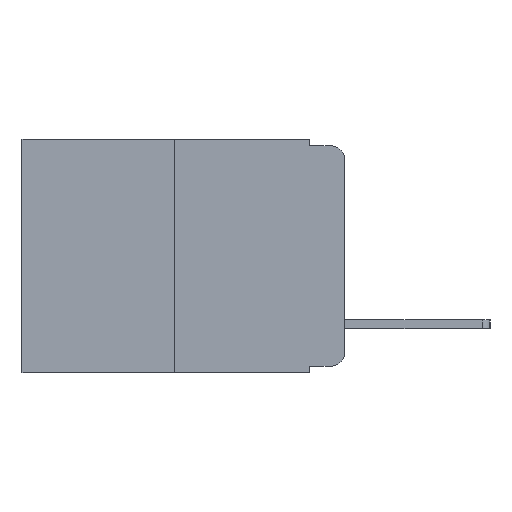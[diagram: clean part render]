
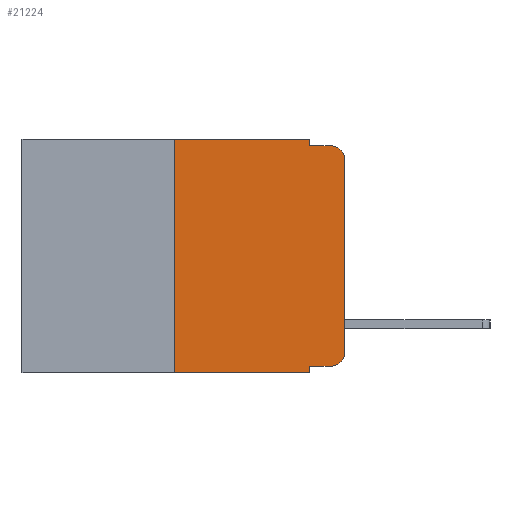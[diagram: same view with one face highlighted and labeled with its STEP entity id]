
A CAD part, left-side view. The second image highlights one B-rep face of the part: STEP entity #21224.
In plain terms, the highlighted planar face has unit normal (-1, 0, 0).
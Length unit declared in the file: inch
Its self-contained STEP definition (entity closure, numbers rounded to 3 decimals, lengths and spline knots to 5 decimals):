
#1038 = VERTEX_POINT ( 'NONE', #17887 ) ;
#1089 = VERTEX_POINT ( 'NONE', #10230 ) ;
#1184 = EDGE_CURVE ( 'NONE', #1038, #3285, #2464, .T. ) ;
#1366 = VERTEX_POINT ( 'NONE', #21364 ) ;
#1428 = EDGE_LOOP ( 'NONE', ( #6493, #21380, #1842, #4576, #2442, #1454, #11451, #9322, #11807, #7376 ) ) ;
#1454 = ORIENTED_EDGE ( 'NONE', *, *, #2565, .F. ) ;
#1701 = CIRCLE ( 'NONE', #21722, 0.02 ) ;
#1842 = ORIENTED_EDGE ( 'NONE', *, *, #2498, .F. ) ;
#1847 = EDGE_CURVE ( 'NONE', #9586, #7723, #10729, .T. ) ;
#2425 = EDGE_CURVE ( 'NONE', #1366, #1089, #13126, .T. ) ;
#2428 = EDGE_CURVE ( 'NONE', #1089, #21960, #3283, .T. ) ;
#2442 = ORIENTED_EDGE ( 'NONE', *, *, #1184, .F. ) ;
#2464 = LINE ( 'NONE', #22741, #12940 ) ;
#2498 = EDGE_CURVE ( 'NONE', #7603, #21960, #6714, .T. ) ;
#2534 = EDGE_CURVE ( 'NONE', #3285, #7603, #14385, .T. ) ;
#2565 = EDGE_CURVE ( 'NONE', #9586, #1038, #3569, .T. ) ;
#2567 = EDGE_CURVE ( 'NONE', #15228, #7723, #12837, .T. ) ;
#2607 = EDGE_CURVE ( 'NONE', #15228, #16718, #13386, .T. ) ;
#2643 = EDGE_CURVE ( 'NONE', #16718, #1366, #1701, .T. ) ;
#2973 = VECTOR ( 'NONE', #13992, 39.37008 ) ;
#3014 = DIRECTION ( 'NONE',  ( 0., 0., -1. ) ) ;
#3036 = AXIS2_PLACEMENT_3D ( 'NONE', #14989, #4194, #16692 ) ;
#3182 = DIRECTION ( 'NONE',  ( 0., -1., 0. ) ) ;
#3283 = CIRCLE ( 'NONE', #3036, 0.02 ) ;
#3285 = VERTEX_POINT ( 'NONE', #9413 ) ;
#3569 = LINE ( 'NONE', #15731, #17275 ) ;
#3944 = CARTESIAN_POINT ( 'NONE',  ( 0., 0.051, -0.343 ) ) ;
#3956 = DIRECTION ( 'NONE',  ( 0., -1., 0. ) ) ;
#4105 = DIRECTION ( 'NONE',  ( 0., 0., 1. ) ) ;
#4194 = DIRECTION ( 'NONE',  ( -1., 0., 0. ) ) ;
#4576 = ORIENTED_EDGE ( 'NONE', *, *, #2534, .F. ) ;
#5427 = VECTOR ( 'NONE', #18516, 39.37008 ) ;
#6493 = ORIENTED_EDGE ( 'NONE', *, *, #2425, .T. ) ;
#6714 = LINE ( 'NONE', #12219, #5427 ) ;
#7376 = ORIENTED_EDGE ( 'NONE', *, *, #2643, .T. ) ;
#7422 = CARTESIAN_POINT ( 'NONE',  ( 0., 0.02, -0.313 ) ) ;
#7603 = VERTEX_POINT ( 'NONE', #9153 ) ;
#7723 = VERTEX_POINT ( 'NONE', #3944 ) ;
#8448 = CARTESIAN_POINT ( 'NONE',  ( 0., 0.02, -0.333 ) ) ;
#8639 = FACE_OUTER_BOUND ( 'NONE', #1428, .T. ) ;
#9153 = CARTESIAN_POINT ( 'NONE',  ( 0., 0.051, -0.01 ) ) ;
#9285 = DIRECTION ( 'NONE',  ( 0., 0., -1. ) ) ;
#9322 = ORIENTED_EDGE ( 'NONE', *, *, #2567, .F. ) ;
#9349 = VECTOR ( 'NONE', #3014, 39.37008 ) ;
#9413 = CARTESIAN_POINT ( 'NONE',  ( 0., 0.051, 0. ) ) ;
#9586 = VERTEX_POINT ( 'NONE', #14764 ) ;
#10230 = CARTESIAN_POINT ( 'NONE',  ( 0., 0., -0.03 ) ) ;
#10495 = DIRECTION ( 'NONE',  ( 0., 0., -1. ) ) ;
#10729 = LINE ( 'NONE', #13162, #22814 ) ;
#10881 = DIRECTION ( 'NONE',  ( 0., -1., 0. ) ) ;
#11043 = CARTESIAN_POINT ( 'NONE',  ( 0., 0.051, -0.333 ) ) ;
#11451 = ORIENTED_EDGE ( 'NONE', *, *, #1847, .T. ) ;
#11807 = ORIENTED_EDGE ( 'NONE', *, *, #2607, .T. ) ;
#12219 = CARTESIAN_POINT ( 'NONE',  ( 0., 0.051, -0.01 ) ) ;
#12837 = LINE ( 'NONE', #22174, #2973 ) ;
#12940 = VECTOR ( 'NONE', #3182, 39.37008 ) ;
#13126 = LINE ( 'NONE', #18239, #17032 ) ;
#13162 = CARTESIAN_POINT ( 'NONE',  ( 0., 0.473, -0.343 ) ) ;
#13386 = LINE ( 'NONE', #19127, #16234 ) ;
#13992 = DIRECTION ( 'NONE',  ( 0., 0., -1. ) ) ;
#14344 = CARTESIAN_POINT ( 'NONE',  ( 0., 0.02, -0.01 ) ) ;
#14385 = LINE ( 'NONE', #20501, #9349 ) ;
#14764 = CARTESIAN_POINT ( 'NONE',  ( 0., 0.25, -0.343 ) ) ;
#14989 = CARTESIAN_POINT ( 'NONE',  ( 0., 0.02, -0.03 ) ) ;
#15228 = VERTEX_POINT ( 'NONE', #11043 ) ;
#15731 = CARTESIAN_POINT ( 'NONE',  ( 0., 0.25, 0. ) ) ;
#16234 = VECTOR ( 'NONE', #10881, 39.37008 ) ;
#16692 = DIRECTION ( 'NONE',  ( 0., 0., -1. ) ) ;
#16718 = VERTEX_POINT ( 'NONE', #8448 ) ;
#17032 = VECTOR ( 'NONE', #4105, 39.37008 ) ;
#17275 = VECTOR ( 'NONE', #17395, 39.37008 ) ;
#17395 = DIRECTION ( 'NONE',  ( 0., 0., 1. ) ) ;
#17887 = CARTESIAN_POINT ( 'NONE',  ( 0., 0.25, 0. ) ) ;
#17923 = AXIS2_PLACEMENT_3D ( 'NONE', #20246, #20391, #10495 ) ;
#18239 = CARTESIAN_POINT ( 'NONE',  ( 0., 0., 0. ) ) ;
#18516 = DIRECTION ( 'NONE',  ( 0., -1., 0. ) ) ;
#18760 = PLANE ( 'NONE',  #17923 ) ;
#19127 = CARTESIAN_POINT ( 'NONE',  ( 0., 0.051, -0.333 ) ) ;
#19269 = DIRECTION ( 'NONE',  ( -1., 0., 0. ) ) ;
#20246 = CARTESIAN_POINT ( 'NONE',  ( 0., 0.473, 0. ) ) ;
#20391 = DIRECTION ( 'NONE',  ( 1., 0., 0. ) ) ;
#20501 = CARTESIAN_POINT ( 'NONE',  ( 0., 0.051, 0. ) ) ;
#21224 = ADVANCED_FACE ( 'NONE', ( #8639 ), #18760, .F. ) ;
#21364 = CARTESIAN_POINT ( 'NONE',  ( 0., 0., -0.313 ) ) ;
#21380 = ORIENTED_EDGE ( 'NONE', *, *, #2428, .T. ) ;
#21722 = AXIS2_PLACEMENT_3D ( 'NONE', #7422, #19269, #9285 ) ;
#21960 = VERTEX_POINT ( 'NONE', #14344 ) ;
#22174 = CARTESIAN_POINT ( 'NONE',  ( 0., 0.051, 0. ) ) ;
#22741 = CARTESIAN_POINT ( 'NONE',  ( 0., 0.473, 0. ) ) ;
#22814 = VECTOR ( 'NONE', #3956, 39.37008 ) ;
